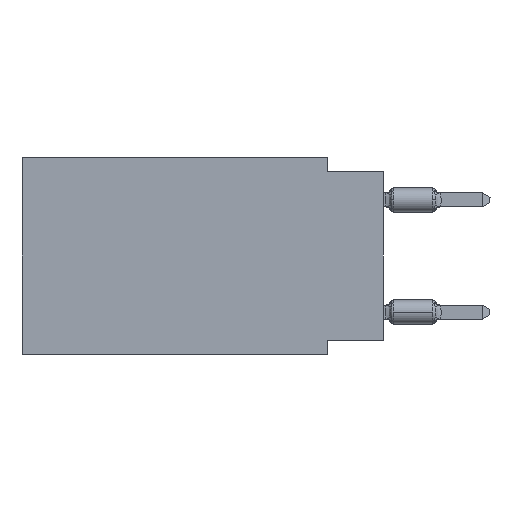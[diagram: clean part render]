
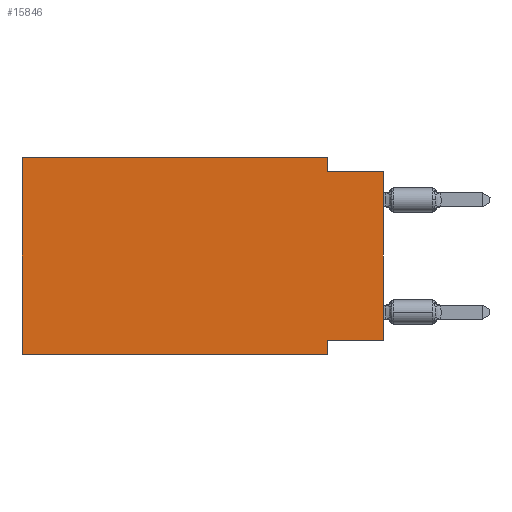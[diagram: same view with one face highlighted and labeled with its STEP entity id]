
A CAD part, left-side view. The second image highlights one B-rep face of the part: STEP entity #15846.
In plain terms, the highlighted planar face has unit normal (-1, 0, 0).
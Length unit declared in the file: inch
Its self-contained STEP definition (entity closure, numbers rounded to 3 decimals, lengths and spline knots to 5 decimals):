
#1510 = EDGE_CURVE ( 'NONE', #13062, #22379, #34783, .T. ) ;
#2463 = DIRECTION ( 'NONE',  ( 0., -1., 0. ) ) ;
#2872 = ORIENTED_EDGE ( 'NONE', *, *, #31599, .F. ) ;
#3913 = DIRECTION ( 'NONE',  ( 0., 0., 1. ) ) ;
#4385 = FACE_OUTER_BOUND ( 'NONE', #55029, .T. ) ;
#5727 = VERTEX_POINT ( 'NONE', #30583 ) ;
#6328 = VECTOR ( 'NONE', #30420, 39.37008 ) ;
#6621 = VERTEX_POINT ( 'NONE', #34458 ) ;
#8320 = ORIENTED_EDGE ( 'NONE', *, *, #15050, .T. ) ;
#9883 = LINE ( 'NONE', #13901, #23116 ) ;
#11557 = CARTESIAN_POINT ( 'NONE',  ( 0., 0., -0.325 ) ) ;
#11849 = CARTESIAN_POINT ( 'NONE',  ( 0., 0., -0.025 ) ) ;
#13062 = VERTEX_POINT ( 'NONE', #43842 ) ;
#13699 = DIRECTION ( 'NONE',  ( 0., 1., 0. ) ) ;
#13901 = CARTESIAN_POINT ( 'NONE',  ( 0., 0.1, 0. ) ) ;
#14217 = DIRECTION ( 'NONE',  ( 0., 0., -1. ) ) ;
#14981 = VECTOR ( 'NONE', #2463, 39.37008 ) ;
#15050 = EDGE_CURVE ( 'NONE', #33149, #28807, #33863, .T. ) ;
#15583 = ORIENTED_EDGE ( 'NONE', *, *, #35025, .F. ) ;
#15846 = ADVANCED_FACE ( 'NONE', ( #4385 ), #46684, .F. ) ;
#16386 = ORIENTED_EDGE ( 'NONE', *, *, #17987, .F. ) ;
#17460 = VECTOR ( 'NONE', #3913, 39.37008 ) ;
#17987 = EDGE_CURVE ( 'NONE', #6621, #34881, #18861, .T. ) ;
#18052 = VECTOR ( 'NONE', #20233, 39.37008 ) ;
#18267 = DIRECTION ( 'NONE',  ( 1., 0., 0. ) ) ;
#18332 = CARTESIAN_POINT ( 'NONE',  ( 0., 0., -0.325 ) ) ;
#18861 = LINE ( 'NONE', #56518, #37274 ) ;
#20233 = DIRECTION ( 'NONE',  ( 0., 0., 1. ) ) ;
#22379 = VERTEX_POINT ( 'NONE', #47899 ) ;
#22416 = CARTESIAN_POINT ( 'NONE',  ( 0., 0.645, 0. ) ) ;
#23116 = VECTOR ( 'NONE', #32139, 39.37008 ) ;
#24473 = EDGE_CURVE ( 'NONE', #33149, #6621, #56598, .T. ) ;
#25371 = EDGE_CURVE ( 'NONE', #5727, #34881, #30597, .T. ) ;
#26215 = AXIS2_PLACEMENT_3D ( 'NONE', #28493, #18267, #55924 ) ;
#27787 = VECTOR ( 'NONE', #44947, 39.37008 ) ;
#28493 = CARTESIAN_POINT ( 'NONE',  ( 0., 0.645, 0. ) ) ;
#28807 = VERTEX_POINT ( 'NONE', #36345 ) ;
#29182 = CARTESIAN_POINT ( 'NONE',  ( 0., 0.1, -0.025 ) ) ;
#30420 = DIRECTION ( 'NONE',  ( 0., -1., 0. ) ) ;
#30583 = CARTESIAN_POINT ( 'NONE',  ( 0., 0.645, -0.35 ) ) ;
#30597 = LINE ( 'NONE', #59545, #14981 ) ;
#31059 = CARTESIAN_POINT ( 'NONE',  ( 0., 0.645, 0. ) ) ;
#31599 = EDGE_CURVE ( 'NONE', #5727, #13062, #46193, .T. ) ;
#32139 = DIRECTION ( 'NONE',  ( 0., 0., -1. ) ) ;
#33149 = VERTEX_POINT ( 'NONE', #11557 ) ;
#33863 = LINE ( 'NONE', #43728, #18052 ) ;
#34458 = CARTESIAN_POINT ( 'NONE',  ( 0., 0.1, -0.325 ) ) ;
#34783 = LINE ( 'NONE', #31059, #27787 ) ;
#34881 = VERTEX_POINT ( 'NONE', #39955 ) ;
#34917 = ORIENTED_EDGE ( 'NONE', *, *, #1510, .F. ) ;
#35019 = LINE ( 'NONE', #11849, #6328 ) ;
#35025 = EDGE_CURVE ( 'NONE', #48772, #28807, #35019, .T. ) ;
#36083 = ORIENTED_EDGE ( 'NONE', *, *, #41547, .F. ) ;
#36345 = CARTESIAN_POINT ( 'NONE',  ( 0., 0., -0.025 ) ) ;
#37274 = VECTOR ( 'NONE', #14217, 39.37008 ) ;
#39955 = CARTESIAN_POINT ( 'NONE',  ( 0., 0.1, -0.35 ) ) ;
#41547 = EDGE_CURVE ( 'NONE', #22379, #48772, #9883, .T. ) ;
#43728 = CARTESIAN_POINT ( 'NONE',  ( 0., 0., 0. ) ) ;
#43842 = CARTESIAN_POINT ( 'NONE',  ( 0., 0.645, 0. ) ) ;
#44947 = DIRECTION ( 'NONE',  ( 0., -1., 0. ) ) ;
#46193 = LINE ( 'NONE', #22416, #17460 ) ;
#46684 = PLANE ( 'NONE',  #26215 ) ;
#47899 = CARTESIAN_POINT ( 'NONE',  ( 0., 0.1, 0. ) ) ;
#48772 = VERTEX_POINT ( 'NONE', #29182 ) ;
#51379 = VECTOR ( 'NONE', #13699, 39.37008 ) ;
#51729 = ORIENTED_EDGE ( 'NONE', *, *, #25371, .T. ) ;
#55029 = EDGE_LOOP ( 'NONE', ( #8320, #15583, #36083, #34917, #2872, #51729, #16386, #60392 ) ) ;
#55924 = DIRECTION ( 'NONE',  ( 0., 0., -1. ) ) ;
#56518 = CARTESIAN_POINT ( 'NONE',  ( 0., 0.1, -0.35 ) ) ;
#56598 = LINE ( 'NONE', #18332, #51379 ) ;
#59545 = CARTESIAN_POINT ( 'NONE',  ( 0., 0.645, -0.35 ) ) ;
#60392 = ORIENTED_EDGE ( 'NONE', *, *, #24473, .F. ) ;
